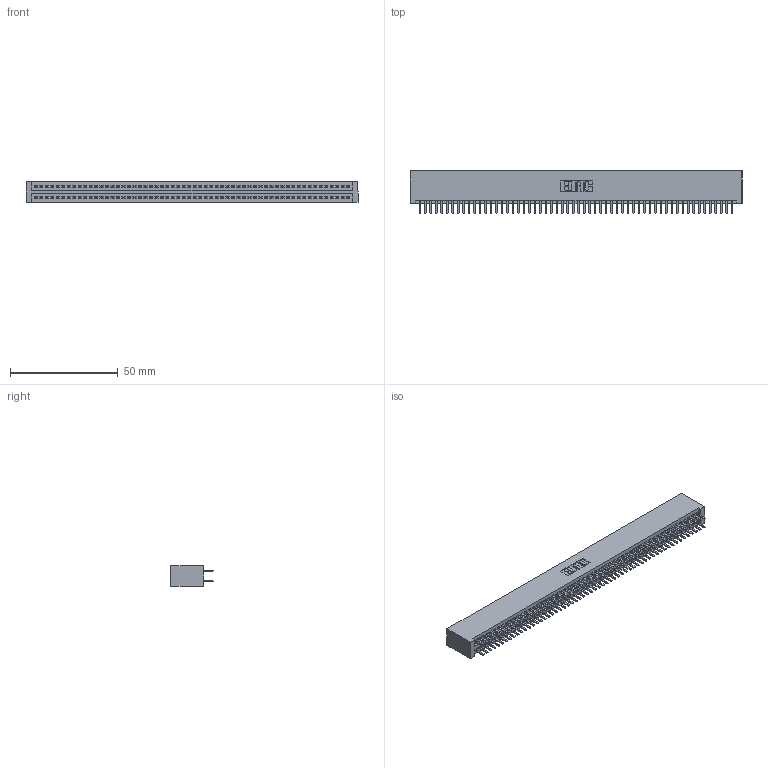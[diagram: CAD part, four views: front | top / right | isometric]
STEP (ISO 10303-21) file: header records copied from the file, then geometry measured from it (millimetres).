
FILE_DESCRIPTION (( 'STEP AP203' ), '1' );
FILE_NAME ('395-116-520-201.STEP', '2018-12-01T20:50:26', ( '' ), ( '' ), 'SwSTEP 2.0', 'SolidWorks 2016', '' );
FILE_SCHEMA (( 'CONFIG_CONTROL_DESIGN' ));
Length unit declared in the file: inch
Products named in the file (3): 345-292-001_345-293-120; 395-116-520-201; 345 Part_No Mounting Lugs
Assembly tree (117 placements, depth 2):
  395-116-520-201
    345 Part_No Mounting Lugs
    345-292-001_345-293-120  x116
Bounding box: 153.92 x 19.68 x 9.4 mm (x, y, z)
Volume: 15665.8 mm3; surface area: 23661.3 mm2
Topology: 117 solids, 117 shells, 6382 faces, 18529 edges, 12042 vertices
Faces by surface type: plane 4136, cylinder 2246
Entity records: 43191 total; most frequent: CARTESIAN_POINT 7236, ORIENTED_EDGE 7158, DIRECTION 6343, EDGE_CURVE 3579, LINE 3219, VECTOR 3219, VERTEX_POINT 2382, AXIS2_PLACEMENT_3D 1562
